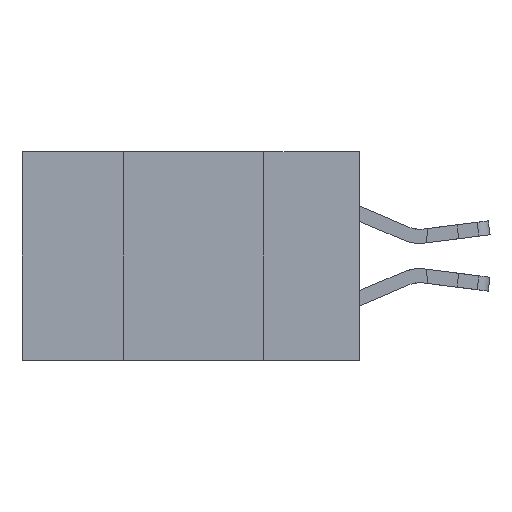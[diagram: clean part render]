
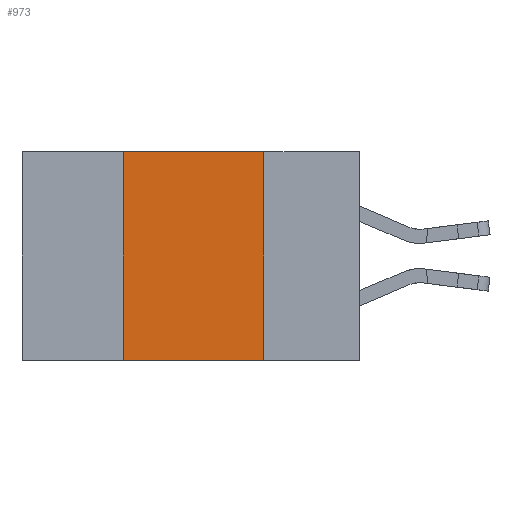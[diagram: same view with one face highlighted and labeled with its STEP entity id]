
A CAD part, left-side view. The second image highlights one B-rep face of the part: STEP entity #973.
In plain terms, the highlighted planar face has unit normal (-1, 0, 0).
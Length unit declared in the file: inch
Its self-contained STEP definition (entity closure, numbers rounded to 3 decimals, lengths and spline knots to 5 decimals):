
#162 = VECTOR ( 'NONE', #13310, 39.37008 ) ;
#225 = CARTESIAN_POINT ( 'NONE',  ( 0., 0.17, 0. ) ) ;
#231 = CARTESIAN_POINT ( 'NONE',  ( 0., 0.42, 0. ) ) ;
#973 = ADVANCED_FACE ( 'NONE', ( #11015 ), #22477, .F. ) ;
#1245 = VECTOR ( 'NONE', #19184, 39.37008 ) ;
#1596 = CARTESIAN_POINT ( 'NONE',  ( 0., 0.6, 0. ) ) ;
#2038 = EDGE_CURVE ( 'NONE', #3917, #20435, #8343, .T. ) ;
#2102 = VECTOR ( 'NONE', #8733, 39.37008 ) ;
#3261 = ORIENTED_EDGE ( 'NONE', *, *, #17514, .F. ) ;
#3459 = LINE ( 'NONE', #10929, #2102 ) ;
#3917 = VERTEX_POINT ( 'NONE', #231 ) ;
#4030 = LINE ( 'NONE', #13563, #162 ) ;
#6662 = CARTESIAN_POINT ( 'NONE',  ( 0., 0.17, -0.37 ) ) ;
#6720 = ORIENTED_EDGE ( 'NONE', *, *, #2038, .F. ) ;
#7124 = ORIENTED_EDGE ( 'NONE', *, *, #16901, .T. ) ;
#7749 = EDGE_LOOP ( 'NONE', ( #18098, #6720, #3261, #7124 ) ) ;
#8343 = LINE ( 'NONE', #11778, #1245 ) ;
#8733 = DIRECTION ( 'NONE',  ( 0., 0., 1. ) ) ;
#10447 = CARTESIAN_POINT ( 'NONE',  ( 0., 0.42, -0.37 ) ) ;
#10929 = CARTESIAN_POINT ( 'NONE',  ( 0., 0.42, 0. ) ) ;
#11015 = FACE_OUTER_BOUND ( 'NONE', #7749, .T. ) ;
#11778 = CARTESIAN_POINT ( 'NONE',  ( 0., 0.6, 0. ) ) ;
#13272 = DIRECTION ( 'NONE',  ( 0., 0., -1. ) ) ;
#13310 = DIRECTION ( 'NONE',  ( 0., -1., 0. ) ) ;
#13563 = CARTESIAN_POINT ( 'NONE',  ( 0., 0.6, -0.37 ) ) ;
#13638 = VERTEX_POINT ( 'NONE', #10447 ) ;
#14649 = DIRECTION ( 'NONE',  ( 0., 0., -1. ) ) ;
#14815 = AXIS2_PLACEMENT_3D ( 'NONE', #1596, #20023, #14649 ) ;
#16901 = EDGE_CURVE ( 'NONE', #13638, #23013, #4030, .T. ) ;
#17514 = EDGE_CURVE ( 'NONE', #13638, #3917, #3459, .T. ) ;
#18098 = ORIENTED_EDGE ( 'NONE', *, *, #23957, .F. ) ;
#18863 = CARTESIAN_POINT ( 'NONE',  ( 0., 0.17, 0. ) ) ;
#19184 = DIRECTION ( 'NONE',  ( 0., -1., 0. ) ) ;
#20023 = DIRECTION ( 'NONE',  ( 1., 0., 0. ) ) ;
#20435 = VERTEX_POINT ( 'NONE', #18863 ) ;
#22433 = LINE ( 'NONE', #225, #23699 ) ;
#22477 = PLANE ( 'NONE',  #14815 ) ;
#23013 = VERTEX_POINT ( 'NONE', #6662 ) ;
#23699 = VECTOR ( 'NONE', #13272, 39.37008 ) ;
#23957 = EDGE_CURVE ( 'NONE', #20435, #23013, #22433, .T. ) ;
